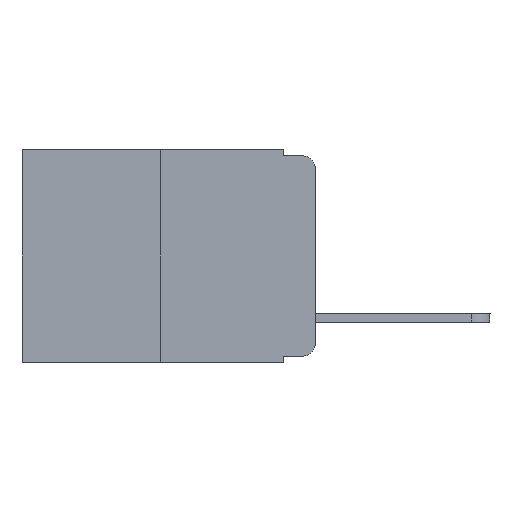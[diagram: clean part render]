
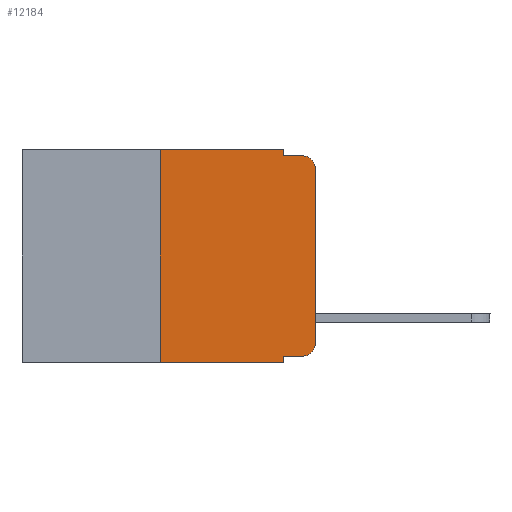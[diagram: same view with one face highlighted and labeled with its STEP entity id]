
A CAD part, left-side view. The second image highlights one B-rep face of the part: STEP entity #12184.
In plain terms, the highlighted planar face has unit normal (-1, 0, 0).
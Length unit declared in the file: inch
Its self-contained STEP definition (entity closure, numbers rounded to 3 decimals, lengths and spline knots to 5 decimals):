
#233 = CARTESIAN_POINT ( 'NONE',  ( 0., 0.051, -0.01 ) ) ;
#322 = VECTOR ( 'NONE', #936, 39.37008 ) ;
#412 = CIRCLE ( 'NONE', #4908, 0.02 ) ;
#491 = DIRECTION ( 'NONE',  ( 0., -1., 0. ) ) ;
#494 = ORIENTED_EDGE ( 'NONE', *, *, #13392, .F. ) ;
#667 = VERTEX_POINT ( 'NONE', #2017 ) ;
#677 = CARTESIAN_POINT ( 'NONE',  ( 0., 0.051, -0.343 ) ) ;
#936 = DIRECTION ( 'NONE',  ( 0., 0., -1. ) ) ;
#1287 = CARTESIAN_POINT ( 'NONE',  ( 0., 0., -0.313 ) ) ;
#1735 = LINE ( 'NONE', #8281, #15001 ) ;
#1783 = CIRCLE ( 'NONE', #8321, 0.02 ) ;
#1917 = PLANE ( 'NONE',  #4429 ) ;
#2017 = CARTESIAN_POINT ( 'NONE',  ( 0., 0.051, -0.333 ) ) ;
#2357 = DIRECTION ( 'NONE',  ( 1., 0., 0. ) ) ;
#2660 = ORIENTED_EDGE ( 'NONE', *, *, #7747, .F. ) ;
#2904 = VERTEX_POINT ( 'NONE', #12922 ) ;
#2913 = ORIENTED_EDGE ( 'NONE', *, *, #10259, .T. ) ;
#3042 = FACE_OUTER_BOUND ( 'NONE', #9276, .T. ) ;
#3310 = VECTOR ( 'NONE', #3892, 39.37008 ) ;
#3654 = LINE ( 'NONE', #6623, #6315 ) ;
#3816 = VERTEX_POINT ( 'NONE', #677 ) ;
#3819 = LINE ( 'NONE', #10764, #10167 ) ;
#3892 = DIRECTION ( 'NONE',  ( 0., -1., 0. ) ) ;
#4429 = AXIS2_PLACEMENT_3D ( 'NONE', #11060, #2357, #6144 ) ;
#4533 = EDGE_CURVE ( 'NONE', #9660, #9136, #412, .T. ) ;
#4908 = AXIS2_PLACEMENT_3D ( 'NONE', #11158, #16450, #9991 ) ;
#4952 = CARTESIAN_POINT ( 'NONE',  ( 0., 0.02, -0.01 ) ) ;
#5301 = CARTESIAN_POINT ( 'NONE',  ( 0., 0.051, -0.01 ) ) ;
#5303 = ORIENTED_EDGE ( 'NONE', *, *, #13947, .T. ) ;
#5598 = DIRECTION ( 'NONE',  ( 0., -1., 0. ) ) ;
#5810 = ORIENTED_EDGE ( 'NONE', *, *, #8932, .T. ) ;
#5870 = LINE ( 'NONE', #7424, #322 ) ;
#5981 = LINE ( 'NONE', #9036, #3310 ) ;
#6144 = DIRECTION ( 'NONE',  ( 0., 0., -1. ) ) ;
#6315 = VECTOR ( 'NONE', #15783, 39.37008 ) ;
#6623 = CARTESIAN_POINT ( 'NONE',  ( 0., 0.051, 0. ) ) ;
#6697 = VECTOR ( 'NONE', #12104, 39.37008 ) ;
#6911 = CARTESIAN_POINT ( 'NONE',  ( 0., 0.051, 0. ) ) ;
#7217 = EDGE_CURVE ( 'NONE', #16448, #11356, #12806, .T. ) ;
#7424 = CARTESIAN_POINT ( 'NONE',  ( 0., 0.051, 0. ) ) ;
#7747 = EDGE_CURVE ( 'NONE', #11356, #13475, #3819, .T. ) ;
#8135 = EDGE_CURVE ( 'NONE', #13475, #15839, #5870, .T. ) ;
#8281 = CARTESIAN_POINT ( 'NONE',  ( 0., 0.473, -0.343 ) ) ;
#8321 = AXIS2_PLACEMENT_3D ( 'NONE', #8867, #9336, #14501 ) ;
#8426 = ORIENTED_EDGE ( 'NONE', *, *, #10971, .T. ) ;
#8610 = LINE ( 'NONE', #9284, #12513 ) ;
#8867 = CARTESIAN_POINT ( 'NONE',  ( 0., 0.02, -0.313 ) ) ;
#8932 = EDGE_CURVE ( 'NONE', #16448, #3816, #1735, .T. ) ;
#9036 = CARTESIAN_POINT ( 'NONE',  ( 0., 0.051, -0.333 ) ) ;
#9063 = DIRECTION ( 'NONE',  ( 0., -1., 0. ) ) ;
#9136 = VERTEX_POINT ( 'NONE', #4952 ) ;
#9276 = EDGE_LOOP ( 'NONE', ( #8426, #9319, #494, #13271, #2660, #15266, #5810, #14793, #2913, #5303 ) ) ;
#9284 = CARTESIAN_POINT ( 'NONE',  ( 0., 0., 0. ) ) ;
#9319 = ORIENTED_EDGE ( 'NONE', *, *, #4533, .T. ) ;
#9336 = DIRECTION ( 'NONE',  ( -1., 0., 0. ) ) ;
#9660 = VERTEX_POINT ( 'NONE', #16708 ) ;
#9991 = DIRECTION ( 'NONE',  ( 0., 0., -1. ) ) ;
#10167 = VECTOR ( 'NONE', #491, 39.37008 ) ;
#10259 = EDGE_CURVE ( 'NONE', #667, #2904, #5981, .T. ) ;
#10414 = CARTESIAN_POINT ( 'NONE',  ( 0., 0.25, -0.343 ) ) ;
#10764 = CARTESIAN_POINT ( 'NONE',  ( 0., 0.473, 0. ) ) ;
#10822 = CARTESIAN_POINT ( 'NONE',  ( 0., 0.25, 0. ) ) ;
#10934 = VERTEX_POINT ( 'NONE', #1287 ) ;
#10971 = EDGE_CURVE ( 'NONE', #10934, #9660, #8610, .T. ) ;
#11060 = CARTESIAN_POINT ( 'NONE',  ( 0., 0.473, 0. ) ) ;
#11158 = CARTESIAN_POINT ( 'NONE',  ( 0., 0.02, -0.03 ) ) ;
#11356 = VERTEX_POINT ( 'NONE', #15730 ) ;
#11907 = EDGE_CURVE ( 'NONE', #667, #3816, #3654, .T. ) ;
#12104 = DIRECTION ( 'NONE',  ( 0., 0., 1. ) ) ;
#12184 = ADVANCED_FACE ( 'NONE', ( #3042 ), #1917, .F. ) ;
#12513 = VECTOR ( 'NONE', #13109, 39.37008 ) ;
#12806 = LINE ( 'NONE', #10822, #6697 ) ;
#12922 = CARTESIAN_POINT ( 'NONE',  ( 0., 0.02, -0.333 ) ) ;
#13109 = DIRECTION ( 'NONE',  ( 0., 0., 1. ) ) ;
#13271 = ORIENTED_EDGE ( 'NONE', *, *, #8135, .F. ) ;
#13392 = EDGE_CURVE ( 'NONE', #15839, #9136, #15982, .T. ) ;
#13475 = VERTEX_POINT ( 'NONE', #6911 ) ;
#13947 = EDGE_CURVE ( 'NONE', #2904, #10934, #1783, .T. ) ;
#14501 = DIRECTION ( 'NONE',  ( 0., 0., -1. ) ) ;
#14793 = ORIENTED_EDGE ( 'NONE', *, *, #11907, .F. ) ;
#15001 = VECTOR ( 'NONE', #5598, 39.37008 ) ;
#15153 = VECTOR ( 'NONE', #9063, 39.37008 ) ;
#15266 = ORIENTED_EDGE ( 'NONE', *, *, #7217, .F. ) ;
#15730 = CARTESIAN_POINT ( 'NONE',  ( 0., 0.25, 0. ) ) ;
#15783 = DIRECTION ( 'NONE',  ( 0., 0., -1. ) ) ;
#15839 = VERTEX_POINT ( 'NONE', #233 ) ;
#15982 = LINE ( 'NONE', #5301, #15153 ) ;
#16448 = VERTEX_POINT ( 'NONE', #10414 ) ;
#16450 = DIRECTION ( 'NONE',  ( -1., 0., 0. ) ) ;
#16708 = CARTESIAN_POINT ( 'NONE',  ( 0., 0., -0.03 ) ) ;
